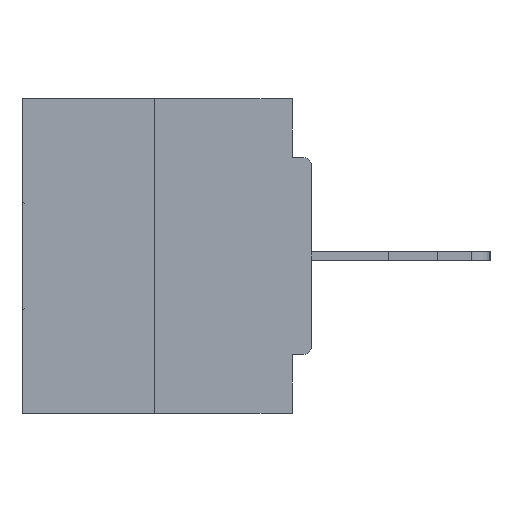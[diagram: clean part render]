
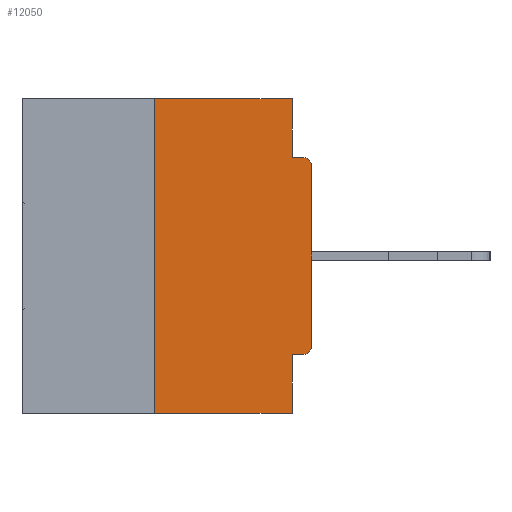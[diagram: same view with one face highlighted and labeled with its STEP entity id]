
A CAD part, left-side view. The second image highlights one B-rep face of the part: STEP entity #12050.
In plain terms, the highlighted planar face has unit normal (-1, 0, 0).
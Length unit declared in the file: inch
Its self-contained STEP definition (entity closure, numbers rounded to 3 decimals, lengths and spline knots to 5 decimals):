
#706 = VERTEX_POINT ( 'NONE', #20072 ) ;
#1097 = AXIS2_PLACEMENT_3D ( 'NONE', #27517, #10681, #13481 ) ;
#1661 = CARTESIAN_POINT ( 'NONE',  ( 0., 0.031, 0. ) ) ;
#2002 = LINE ( 'NONE', #24454, #12186 ) ;
#2596 = DIRECTION ( 'NONE',  ( 0., 0., -1. ) ) ;
#3428 = EDGE_CURVE ( 'NONE', #18544, #10825, #20792, .T. ) ;
#3748 = VECTOR ( 'NONE', #14111, 39.37008 ) ;
#4613 = DIRECTION ( 'NONE',  ( 0., -1., 0. ) ) ;
#4620 = DIRECTION ( 'NONE',  ( -1., 0., 0. ) ) ;
#4652 = LINE ( 'NONE', #8502, #11248 ) ;
#4867 = CARTESIAN_POINT ( 'NONE',  ( 0., 0., -0.4065 ) ) ;
#5977 = LINE ( 'NONE', #14222, #3748 ) ;
#6084 = LINE ( 'NONE', #4867, #25884 ) ;
#7134 = AXIS2_PLACEMENT_3D ( 'NONE', #13684, #30169, #2596 ) ;
#7206 = VERTEX_POINT ( 'NONE', #15139 ) ;
#7386 = EDGE_CURVE ( 'NONE', #10825, #11304, #8861, .T. ) ;
#7416 = ORIENTED_EDGE ( 'NONE', *, *, #10850, .T. ) ;
#7571 = VECTOR ( 'NONE', #14805, 39.37008 ) ;
#7602 = CARTESIAN_POINT ( 'NONE',  ( 0., 0.015, -0.3915 ) ) ;
#7816 = DIRECTION ( 'NONE',  ( 0., 1., 0. ) ) ;
#8502 = CARTESIAN_POINT ( 'NONE',  ( 0., 0., -0.0935 ) ) ;
#8723 = CARTESIAN_POINT ( 'NONE',  ( 0., 0.031, -0.5 ) ) ;
#8861 = LINE ( 'NONE', #31524, #7571 ) ;
#9829 = CARTESIAN_POINT ( 'NONE',  ( 0., 0., 0. ) ) ;
#9954 = VECTOR ( 'NONE', #4613, 39.37008 ) ;
#10681 = DIRECTION ( 'NONE',  ( -1., 0., 0. ) ) ;
#10825 = VERTEX_POINT ( 'NONE', #19528 ) ;
#10850 = EDGE_CURVE ( 'NONE', #13266, #7206, #20184, .T. ) ;
#11248 = VECTOR ( 'NONE', #25487, 39.37008 ) ;
#11291 = EDGE_CURVE ( 'NONE', #17027, #20055, #2002, .T. ) ;
#11304 = VERTEX_POINT ( 'NONE', #1661 ) ;
#11432 = DIRECTION ( 'NONE',  ( 0., 0., 1. ) ) ;
#11671 = FACE_OUTER_BOUND ( 'NONE', #23764, .T. ) ;
#12050 = ADVANCED_FACE ( 'NONE', ( #11671 ), #21933, .F. ) ;
#12186 = VECTOR ( 'NONE', #21512, 39.37008 ) ;
#12910 = ORIENTED_EDGE ( 'NONE', *, *, #29140, .F. ) ;
#13266 = VERTEX_POINT ( 'NONE', #14240 ) ;
#13375 = ORIENTED_EDGE ( 'NONE', *, *, #14096, .T. ) ;
#13481 = DIRECTION ( 'NONE',  ( 0., 0., -1. ) ) ;
#13684 = CARTESIAN_POINT ( 'NONE',  ( 0., 0.46, 0. ) ) ;
#13731 = ORIENTED_EDGE ( 'NONE', *, *, #11291, .F. ) ;
#13770 = LINE ( 'NONE', #9829, #20413 ) ;
#14096 = EDGE_CURVE ( 'NONE', #29350, #29149, #36211, .T. ) ;
#14111 = DIRECTION ( 'NONE',  ( 0., 0., -1. ) ) ;
#14222 = CARTESIAN_POINT ( 'NONE',  ( 0., 0.031, 0. ) ) ;
#14240 = CARTESIAN_POINT ( 'NONE',  ( 0., 0., -0.1085 ) ) ;
#14629 = VECTOR ( 'NONE', #11432, 39.37008 ) ;
#14805 = DIRECTION ( 'NONE',  ( 0., -1., 0. ) ) ;
#14917 = ORIENTED_EDGE ( 'NONE', *, *, #16750, .T. ) ;
#15139 = CARTESIAN_POINT ( 'NONE',  ( 0., 0.015, -0.0935 ) ) ;
#16504 = CARTESIAN_POINT ( 'NONE',  ( 0., 0., -0.3915 ) ) ;
#16566 = AXIS2_PLACEMENT_3D ( 'NONE', #7602, #4620, #35622 ) ;
#16750 = EDGE_CURVE ( 'NONE', #29149, #13266, #13770, .T. ) ;
#16956 = CARTESIAN_POINT ( 'NONE',  ( 0., 0.25, -0.5 ) ) ;
#17027 = VERTEX_POINT ( 'NONE', #34285 ) ;
#17065 = ORIENTED_EDGE ( 'NONE', *, *, #7386, .F. ) ;
#18544 = VERTEX_POINT ( 'NONE', #16956 ) ;
#18670 = DIRECTION ( 'NONE',  ( 0., 0., 1. ) ) ;
#19528 = CARTESIAN_POINT ( 'NONE',  ( 0., 0.25, 0. ) ) ;
#19812 = CARTESIAN_POINT ( 'NONE',  ( 0., 0.25, 0. ) ) ;
#20055 = VERTEX_POINT ( 'NONE', #8723 ) ;
#20072 = CARTESIAN_POINT ( 'NONE',  ( 0., 0.031, -0.0935 ) ) ;
#20184 = CIRCLE ( 'NONE', #1097, 0.015 ) ;
#20413 = VECTOR ( 'NONE', #18670, 39.37008 ) ;
#20537 = LINE ( 'NONE', #35615, #9954 ) ;
#20792 = LINE ( 'NONE', #19812, #14629 ) ;
#21512 = DIRECTION ( 'NONE',  ( 0., 0., -1. ) ) ;
#21933 = PLANE ( 'NONE',  #7134 ) ;
#23566 = ORIENTED_EDGE ( 'NONE', *, *, #24400, .F. ) ;
#23764 = EDGE_LOOP ( 'NONE', ( #17065, #26744, #36456, #13731, #12910, #13375, #14917, #7416, #23566, #25090 ) ) ;
#24400 = EDGE_CURVE ( 'NONE', #706, #7206, #4652, .T. ) ;
#24454 = CARTESIAN_POINT ( 'NONE',  ( 0., 0.031, -0.5 ) ) ;
#25090 = ORIENTED_EDGE ( 'NONE', *, *, #29996, .F. ) ;
#25487 = DIRECTION ( 'NONE',  ( 0., -1., 0. ) ) ;
#25884 = VECTOR ( 'NONE', #7816, 39.37008 ) ;
#26744 = ORIENTED_EDGE ( 'NONE', *, *, #3428, .F. ) ;
#27517 = CARTESIAN_POINT ( 'NONE',  ( 0., 0.015, -0.1085 ) ) ;
#29140 = EDGE_CURVE ( 'NONE', #29350, #17027, #6084, .T. ) ;
#29149 = VERTEX_POINT ( 'NONE', #16504 ) ;
#29350 = VERTEX_POINT ( 'NONE', #36432 ) ;
#29996 = EDGE_CURVE ( 'NONE', #11304, #706, #5977, .T. ) ;
#30169 = DIRECTION ( 'NONE',  ( 1., 0., 0. ) ) ;
#31524 = CARTESIAN_POINT ( 'NONE',  ( 0., 0.46, 0. ) ) ;
#34285 = CARTESIAN_POINT ( 'NONE',  ( 0., 0.031, -0.4065 ) ) ;
#35584 = EDGE_CURVE ( 'NONE', #18544, #20055, #20537, .T. ) ;
#35615 = CARTESIAN_POINT ( 'NONE',  ( 0., 0.46, -0.5 ) ) ;
#35622 = DIRECTION ( 'NONE',  ( 0., 0., -1. ) ) ;
#36211 = CIRCLE ( 'NONE', #16566, 0.015 ) ;
#36432 = CARTESIAN_POINT ( 'NONE',  ( 0., 0.015, -0.4065 ) ) ;
#36456 = ORIENTED_EDGE ( 'NONE', *, *, #35584, .T. ) ;
